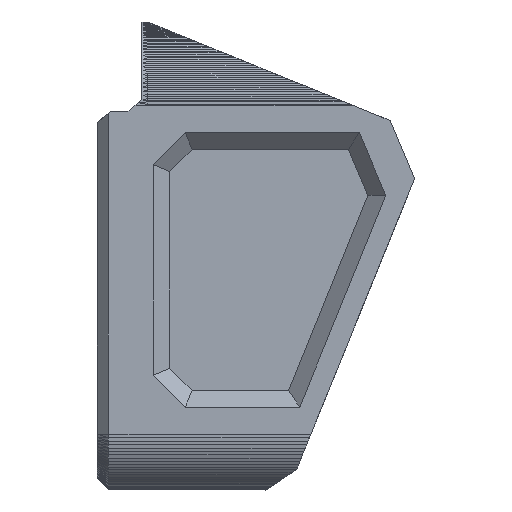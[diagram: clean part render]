
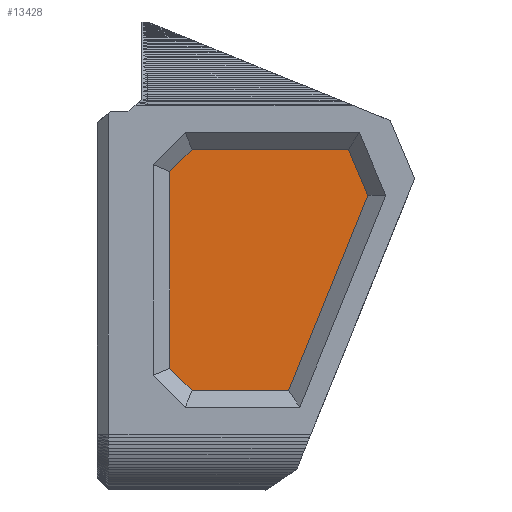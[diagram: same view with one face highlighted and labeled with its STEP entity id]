
A CAD part, left-side view. The second image highlights one B-rep face of the part: STEP entity #13428.
In plain terms, the highlighted planar face has unit normal (-1, 0, 0).
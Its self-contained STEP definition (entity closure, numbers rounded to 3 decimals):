
#752=FACE_OUTER_BOUND('',#1584,.T.);
#1584=EDGE_LOOP('',(#10324,#10325,#10326,#10327,#10328,#10329,#10330));
#2838=LINE('',#21036,#4495);
#2841=LINE('',#21041,#4498);
#2843=LINE('',#21045,#4500);
#2845=LINE('',#21049,#4502);
#2846=LINE('',#21052,#4503);
#2848=LINE('',#21056,#4505);
#2850=LINE('',#21059,#4507);
#4495=VECTOR('',#15843,10.);
#4498=VECTOR('',#15848,10.);
#4500=VECTOR('',#15852,10.);
#4502=VECTOR('',#15856,10.);
#4503=VECTOR('',#15859,10.);
#4505=VECTOR('',#15863,10.);
#4507=VECTOR('',#15867,10.);
#6190=VERTEX_POINT('',#21033);
#6191=VERTEX_POINT('',#21035);
#6192=VERTEX_POINT('',#21039);
#6193=VERTEX_POINT('',#21043);
#6194=VERTEX_POINT('',#21047);
#6195=VERTEX_POINT('',#21051);
#6196=VERTEX_POINT('',#21055);
#7612=EDGE_CURVE('',#6190,#6191,#2838,.T.);
#7615=EDGE_CURVE('',#6192,#6190,#2841,.T.);
#7617=EDGE_CURVE('',#6193,#6192,#2843,.T.);
#7619=EDGE_CURVE('',#6194,#6193,#2845,.T.);
#7620=EDGE_CURVE('',#6191,#6195,#2846,.T.);
#7622=EDGE_CURVE('',#6195,#6196,#2848,.T.);
#7624=EDGE_CURVE('',#6196,#6194,#2850,.T.);
#10324=ORIENTED_EDGE('',*,*,#7617,.F.);
#10325=ORIENTED_EDGE('',*,*,#7619,.F.);
#10326=ORIENTED_EDGE('',*,*,#7624,.F.);
#10327=ORIENTED_EDGE('',*,*,#7622,.F.);
#10328=ORIENTED_EDGE('',*,*,#7620,.F.);
#10329=ORIENTED_EDGE('',*,*,#7612,.F.);
#10330=ORIENTED_EDGE('',*,*,#7615,.F.);
#12614=PLANE('',#14179);
#13428=ADVANCED_FACE('',(#752),#12614,.F.);
#14179=AXIS2_PLACEMENT_3D('',#21060,#15868,#15869);
#15843=DIRECTION('',(0.,0.376,-0.927));
#15848=DIRECTION('',(0.,-0.389,-0.921));
#15852=DIRECTION('',(0.,-1.,0.));
#15856=DIRECTION('',(0.,-0.707,0.707));
#15859=DIRECTION('',(0.,1.,0.));
#15863=DIRECTION('',(0.,0.707,0.707));
#15867=DIRECTION('',(0.,0.,1.));
#15868=DIRECTION('center_axis',(1.,0.,0.));
#15869=DIRECTION('ref_axis',(0.,0.,-1.));
#21033=CARTESIAN_POINT('',(-65.545,-142.718,-155.617));
#21035=CARTESIAN_POINT('',(-65.545,-71.591,-330.783));
#21036=CARTESIAN_POINT('',(-65.545,-142.718,-155.617));
#21039=CARTESIAN_POINT('',(-65.545,-125.229,-114.215));
#21041=CARTESIAN_POINT('',(-65.545,-125.229,-114.215));
#21043=CARTESIAN_POINT('',(-65.545,15.,-114.215));
#21045=CARTESIAN_POINT('',(-65.545,15.,-114.215));
#21047=CARTESIAN_POINT('',(-65.545,35.,-134.215));
#21049=CARTESIAN_POINT('',(-65.545,15.,-114.215));
#21051=CARTESIAN_POINT('',(-65.545,15.,-330.783));
#21052=CARTESIAN_POINT('',(-65.545,-71.591,-330.783));
#21055=CARTESIAN_POINT('',(-65.545,35.,-310.783));
#21056=CARTESIAN_POINT('',(-65.545,15.,-330.783));
#21059=CARTESIAN_POINT('',(-65.545,35.,-134.215));
#21060=CARTESIAN_POINT('Origin',(-65.545,-53.859,-222.499));
